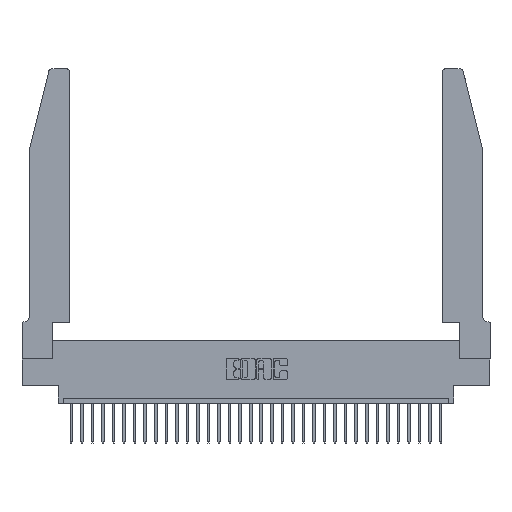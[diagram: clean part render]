
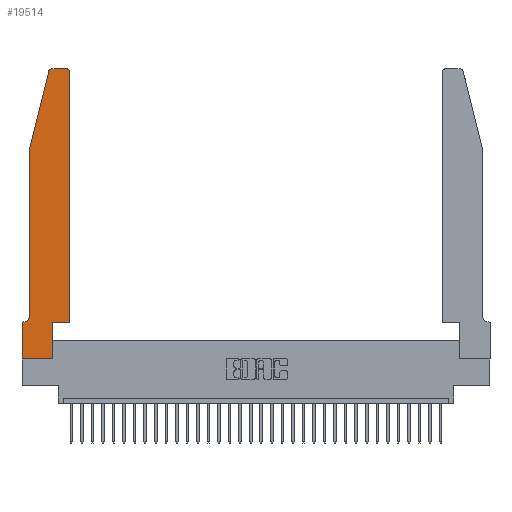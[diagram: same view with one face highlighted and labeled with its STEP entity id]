
A CAD part, top view. The second image highlights one B-rep face of the part: STEP entity #19514.
In plain terms, the highlighted planar face has unit normal (0, 0, 1).
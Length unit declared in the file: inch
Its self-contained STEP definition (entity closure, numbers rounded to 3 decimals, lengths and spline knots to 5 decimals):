
#795 = CARTESIAN_POINT ( 'NONE',  ( 0.0055, 0.42, 0.37 ) ) ;
#818 = DIRECTION ( 'NONE',  ( 1., 0., 0. ) ) ;
#1153 = ORIENTED_EDGE ( 'NONE', *, *, #21610, .T. ) ;
#1296 = ORIENTED_EDGE ( 'NONE', *, *, #5570, .T. ) ;
#1963 = EDGE_CURVE ( 'NONE', #3517, #6465, #18907, .T. ) ;
#2095 = DIRECTION ( 'NONE',  ( 1., 0., 0. ) ) ;
#2588 = AXIS2_PLACEMENT_3D ( 'NONE', #795, #3013, #18585 ) ;
#2748 = VECTOR ( 'NONE', #2095, 39.37008 ) ;
#2924 = AXIS2_PLACEMENT_3D ( 'NONE', #14319, #24542, #29859 ) ;
#3013 = DIRECTION ( 'NONE',  ( 0., 0., -1. ) ) ;
#3122 = ORIENTED_EDGE ( 'NONE', *, *, #1963, .T. ) ;
#3172 = VERTEX_POINT ( 'NONE', #21676 ) ;
#3195 = VERTEX_POINT ( 'NONE', #9453 ) ;
#3239 = CIRCLE ( 'NONE', #2588, 0.07 ) ;
#3434 = VECTOR ( 'NONE', #12590, 39.37008 ) ;
#3517 = VERTEX_POINT ( 'NONE', #12605 ) ;
#3653 = CARTESIAN_POINT ( 'NONE',  ( 0.2865, 0., 0.37 ) ) ;
#4468 = CARTESIAN_POINT ( 'NONE',  ( 0.2605, 2.75, 0.37 ) ) ;
#5493 = CIRCLE ( 'NONE', #2924, 0.03 ) ;
#5570 = EDGE_CURVE ( 'NONE', #22647, #20194, #29754, .T. ) ;
#5938 = ORIENTED_EDGE ( 'NONE', *, *, #6278, .T. ) ;
#6278 = EDGE_CURVE ( 'NONE', #9007, #3172, #5493, .T. ) ;
#6314 = DIRECTION ( 'NONE',  ( 1., 0., 0. ) ) ;
#6383 = DIRECTION ( 'NONE',  ( 0., -1., 0. ) ) ;
#6399 = LINE ( 'NONE', #24703, #20665 ) ;
#6465 = VERTEX_POINT ( 'NONE', #18440 ) ;
#6629 = CARTESIAN_POINT ( 'NONE',  ( 0., 0., 0.37 ) ) ;
#6901 = CARTESIAN_POINT ( 'NONE',  ( 0.4505, 0.35, 0.37 ) ) ;
#8141 = VECTOR ( 'NONE', #14011, 39.37008 ) ;
#8275 = ORIENTED_EDGE ( 'NONE', *, *, #11569, .T. ) ;
#8305 = CARTESIAN_POINT ( 'NONE',  ( 0.0755, 2., 0.37 ) ) ;
#9007 = VERTEX_POINT ( 'NONE', #15615 ) ;
#9276 = ORIENTED_EDGE ( 'NONE', *, *, #30391, .T. ) ;
#9371 = EDGE_CURVE ( 'NONE', #20194, #3195, #9784, .T. ) ;
#9453 = CARTESIAN_POINT ( 'NONE',  ( 0.4505, 2.72, 0.37 ) ) ;
#9784 = LINE ( 'NONE', #6901, #14550 ) ;
#10036 = CARTESIAN_POINT ( 'NONE',  ( 0.0755, 2., 0.37 ) ) ;
#10946 = VECTOR ( 'NONE', #13434, 39.37008 ) ;
#10955 = VECTOR ( 'NONE', #29613, 39.37008 ) ;
#11056 = AXIS2_PLACEMENT_3D ( 'NONE', #27012, #31889, #6314 ) ;
#11400 = DIRECTION ( 'NONE',  ( 1., 0., 0. ) ) ;
#11417 = AXIS2_PLACEMENT_3D ( 'NONE', #28642, #16042, #818 ) ;
#11569 = EDGE_CURVE ( 'NONE', #23791, #3517, #3239, .T. ) ;
#11937 = CARTESIAN_POINT ( 'NONE',  ( 0.4205, 2.75, 0.37 ) ) ;
#12168 = LINE ( 'NONE', #10036, #3434 ) ;
#12545 = LINE ( 'NONE', #8305, #10955 ) ;
#12590 = DIRECTION ( 'NONE',  ( -0.239, -0.971, 0. ) ) ;
#12605 = CARTESIAN_POINT ( 'NONE',  ( 0.0055, 0.35, 0.37 ) ) ;
#12771 = ORIENTED_EDGE ( 'NONE', *, *, #9371, .T. ) ;
#13434 = DIRECTION ( 'NONE',  ( -1., 0., 0. ) ) ;
#13777 = CARTESIAN_POINT ( 'NONE',  ( 0.0755, 2., 0.37 ) ) ;
#14011 = DIRECTION ( 'NONE',  ( -1., 0., 0. ) ) ;
#14047 = PLANE ( 'NONE',  #11056 ) ;
#14319 = CARTESIAN_POINT ( 'NONE',  ( 0.284, 2.72, 0.37 ) ) ;
#14550 = VECTOR ( 'NONE', #24624, 39.37008 ) ;
#14788 = EDGE_LOOP ( 'NONE', ( #1153, #5938, #18190, #16094, #8275, #3122, #30592, #32673, #9276, #1296, #12771, #23378 ) ) ;
#14952 = EDGE_CURVE ( 'NONE', #25564, #23791, #12545, .T. ) ;
#15582 = EDGE_CURVE ( 'NONE', #32358, #24596, #26384, .T. ) ;
#15615 = CARTESIAN_POINT ( 'NONE',  ( 0.284, 2.75, 0.37 ) ) ;
#16042 = DIRECTION ( 'NONE',  ( 0., 0., 1. ) ) ;
#16092 = EDGE_CURVE ( 'NONE', #3195, #29489, #30693, .T. ) ;
#16094 = ORIENTED_EDGE ( 'NONE', *, *, #14952, .T. ) ;
#16162 = CARTESIAN_POINT ( 'NONE',  ( 0., 0., 0.37 ) ) ;
#17334 = CARTESIAN_POINT ( 'NONE',  ( 0.4505, 0.35, 0.37 ) ) ;
#17372 = CARTESIAN_POINT ( 'NONE',  ( 0.4505, 0.35, 0.37 ) ) ;
#18190 = ORIENTED_EDGE ( 'NONE', *, *, #21456, .T. ) ;
#18440 = CARTESIAN_POINT ( 'NONE',  ( 0., 0.35, 0.37 ) ) ;
#18585 = DIRECTION ( 'NONE',  ( -1., 0., 0. ) ) ;
#18677 = FACE_OUTER_BOUND ( 'NONE', #14788, .T. ) ;
#18907 = LINE ( 'NONE', #19615, #8141 ) ;
#19514 = ADVANCED_FACE ( 'NONE', ( #18677 ), #14047, .T. ) ;
#19587 = EDGE_CURVE ( 'NONE', #6465, #32358, #30912, .T. ) ;
#19615 = CARTESIAN_POINT ( 'NONE',  ( 0.0755, 0.35, 0.37 ) ) ;
#20194 = VERTEX_POINT ( 'NONE', #17372 ) ;
#20665 = VECTOR ( 'NONE', #26465, 39.37008 ) ;
#20983 = VECTOR ( 'NONE', #6383, 39.37008 ) ;
#21456 = EDGE_CURVE ( 'NONE', #3172, #25564, #12168, .T. ) ;
#21610 = EDGE_CURVE ( 'NONE', #29489, #9007, #25233, .T. ) ;
#21676 = CARTESIAN_POINT ( 'NONE',  ( 0.25487, 2.72718, 0.37 ) ) ;
#21738 = CARTESIAN_POINT ( 'NONE',  ( 0.0755, 0.42, 0.37 ) ) ;
#22647 = VERTEX_POINT ( 'NONE', #29555 ) ;
#23378 = ORIENTED_EDGE ( 'NONE', *, *, #16092, .T. ) ;
#23791 = VERTEX_POINT ( 'NONE', #21738 ) ;
#24542 = DIRECTION ( 'NONE',  ( 0., 0., 1. ) ) ;
#24596 = VERTEX_POINT ( 'NONE', #3653 ) ;
#24624 = DIRECTION ( 'NONE',  ( 0., 1., 0. ) ) ;
#24703 = CARTESIAN_POINT ( 'NONE',  ( 0.2865, 0.35, 0.37 ) ) ;
#25233 = LINE ( 'NONE', #4468, #10946 ) ;
#25564 = VERTEX_POINT ( 'NONE', #13777 ) ;
#25962 = VECTOR ( 'NONE', #11400, 39.37008 ) ;
#26384 = LINE ( 'NONE', #6629, #25962 ) ;
#26465 = DIRECTION ( 'NONE',  ( 0., 1., 0. ) ) ;
#27012 = CARTESIAN_POINT ( 'NONE',  ( 0., 0.35, 0.37 ) ) ;
#28642 = CARTESIAN_POINT ( 'NONE',  ( 0.4205, 2.72, 0.37 ) ) ;
#29489 = VERTEX_POINT ( 'NONE', #11937 ) ;
#29555 = CARTESIAN_POINT ( 'NONE',  ( 0.2865, 0.35, 0.37 ) ) ;
#29613 = DIRECTION ( 'NONE',  ( 0., -1., 0. ) ) ;
#29754 = LINE ( 'NONE', #17334, #2748 ) ;
#29859 = DIRECTION ( 'NONE',  ( 1., 0., 0. ) ) ;
#30374 = CARTESIAN_POINT ( 'NONE',  ( 0., 0., 0.37 ) ) ;
#30391 = EDGE_CURVE ( 'NONE', #24596, #22647, #6399, .T. ) ;
#30592 = ORIENTED_EDGE ( 'NONE', *, *, #19587, .T. ) ;
#30693 = CIRCLE ( 'NONE', #11417, 0.03 ) ;
#30912 = LINE ( 'NONE', #16162, #20983 ) ;
#31889 = DIRECTION ( 'NONE',  ( 0., 0., 1. ) ) ;
#32358 = VERTEX_POINT ( 'NONE', #30374 ) ;
#32673 = ORIENTED_EDGE ( 'NONE', *, *, #15582, .T. ) ;
